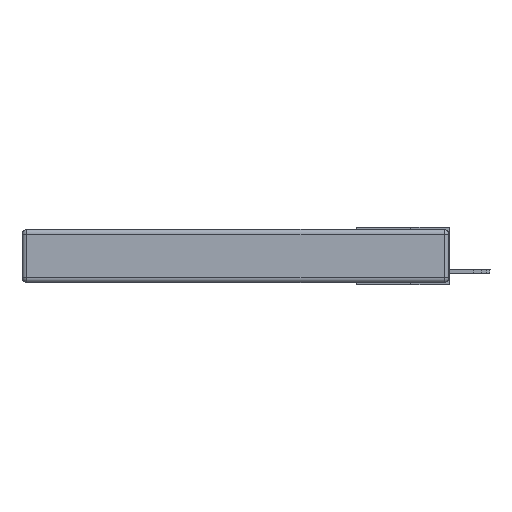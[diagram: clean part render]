
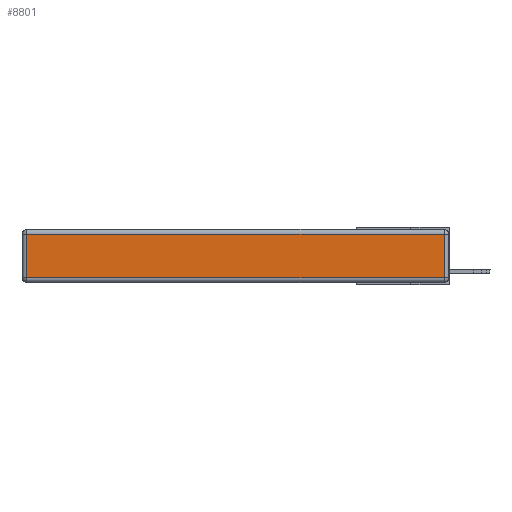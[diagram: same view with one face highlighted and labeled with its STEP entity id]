
A CAD part, left-side view. The second image highlights one B-rep face of the part: STEP entity #8801.
In plain terms, the highlighted planar face has unit normal (-1, 0, 0).
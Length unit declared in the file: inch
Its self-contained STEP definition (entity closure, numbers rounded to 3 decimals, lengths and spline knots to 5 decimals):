
#1228 = VERTEX_POINT ( 'NONE', #20123 ) ;
#2420 = ORIENTED_EDGE ( 'NONE', *, *, #5185, .T. ) ;
#2442 = FACE_OUTER_BOUND ( 'NONE', #14511, .T. ) ;
#2778 = DIRECTION ( 'NONE',  ( 0., -1., 0. ) ) ;
#3136 = LINE ( 'NONE', #3552, #8737 ) ;
#3154 = VERTEX_POINT ( 'NONE', #22284 ) ;
#3323 = DIRECTION ( 'NONE',  ( 0., 1., 0. ) ) ;
#3552 = CARTESIAN_POINT ( 'NONE',  ( 0., 2.72, -0.343 ) ) ;
#3939 = PLANE ( 'NONE',  #5892 ) ;
#4952 = CARTESIAN_POINT ( 'NONE',  ( 0., 2.75, -0.03 ) ) ;
#5185 = EDGE_CURVE ( 'NONE', #3154, #9596, #3136, .T. ) ;
#5643 = DIRECTION ( 'NONE',  ( 0., 0., 1. ) ) ;
#5892 = AXIS2_PLACEMENT_3D ( 'NONE', #20255, #11221, #5643 ) ;
#7724 = VECTOR ( 'NONE', #9389, 39.37008 ) ;
#8737 = VECTOR ( 'NONE', #8948, 39.37008 ) ;
#8801 = ADVANCED_FACE ( 'NONE', ( #2442 ), #3939, .T. ) ;
#8948 = DIRECTION ( 'NONE',  ( 0., 0., -1. ) ) ;
#9389 = DIRECTION ( 'NONE',  ( 0., 0., 1. ) ) ;
#9427 = EDGE_CURVE ( 'NONE', #1228, #19153, #23104, .T. ) ;
#9596 = VERTEX_POINT ( 'NONE', #20863 ) ;
#10199 = CARTESIAN_POINT ( 'NONE',  ( 0., 0.03, -0.03 ) ) ;
#11221 = DIRECTION ( 'NONE',  ( -1., 0., 0. ) ) ;
#11663 = LINE ( 'NONE', #13578, #20820 ) ;
#13578 = CARTESIAN_POINT ( 'NONE',  ( 0., 0., -0.313 ) ) ;
#14055 = VECTOR ( 'NONE', #3323, 39.37008 ) ;
#14511 = EDGE_LOOP ( 'NONE', ( #22025, #19930, #20684, #2420 ) ) ;
#15373 = EDGE_CURVE ( 'NONE', #9596, #1228, #11663, .T. ) ;
#19153 = VERTEX_POINT ( 'NONE', #10199 ) ;
#19930 = ORIENTED_EDGE ( 'NONE', *, *, #9427, .T. ) ;
#20123 = CARTESIAN_POINT ( 'NONE',  ( 0., 0.03, -0.313 ) ) ;
#20255 = CARTESIAN_POINT ( 'NONE',  ( 0., 0., -0.343 ) ) ;
#20684 = ORIENTED_EDGE ( 'NONE', *, *, #21216, .T. ) ;
#20820 = VECTOR ( 'NONE', #2778, 39.37008 ) ;
#20863 = CARTESIAN_POINT ( 'NONE',  ( 0., 2.72, -0.313 ) ) ;
#21216 = EDGE_CURVE ( 'NONE', #19153, #3154, #21465, .T. ) ;
#21465 = LINE ( 'NONE', #4952, #14055 ) ;
#22025 = ORIENTED_EDGE ( 'NONE', *, *, #15373, .T. ) ;
#22284 = CARTESIAN_POINT ( 'NONE',  ( 0., 2.72, -0.03 ) ) ;
#22286 = CARTESIAN_POINT ( 'NONE',  ( 0., 0.03, -0.343 ) ) ;
#23104 = LINE ( 'NONE', #22286, #7724 ) ;
